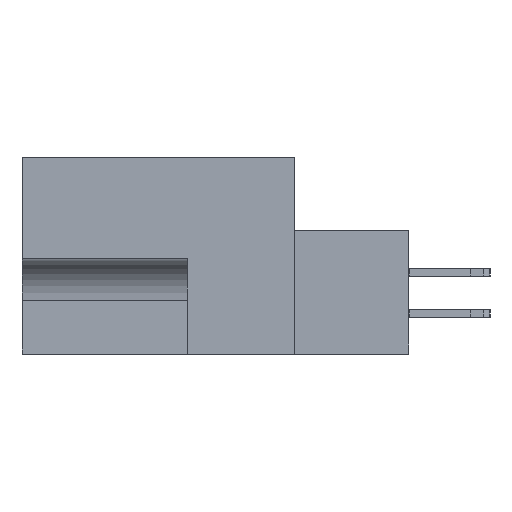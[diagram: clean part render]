
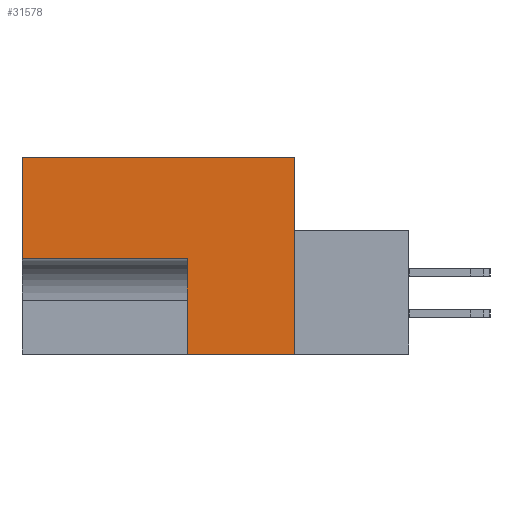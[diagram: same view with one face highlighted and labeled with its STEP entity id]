
A CAD part, left-side view. The second image highlights one B-rep face of the part: STEP entity #31578.
In plain terms, the highlighted planar face has unit normal (-1, 0, 0).
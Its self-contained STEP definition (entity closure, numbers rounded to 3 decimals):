
#2270 = FACE_OUTER_BOUND ( 'NONE', #22167, .T. ) ;
#3450 = ORIENTED_EDGE ( 'NONE', *, *, #34992, .F. ) ;
#3688 = DIRECTION ( 'NONE',  ( 0., 0., 1. ) ) ;
#6347 = DIRECTION ( 'NONE',  ( 1., 0., 0. ) ) ;
#6466 = EDGE_CURVE ( 'NONE', #24307, #24224, #41106, .T. ) ;
#7853 = ORIENTED_EDGE ( 'NONE', *, *, #50835, .F. ) ;
#8285 = CARTESIAN_POINT ( 'NONE',  ( 0., 0., -15.088 ) ) ;
#8500 = CARTESIAN_POINT ( 'NONE',  ( 0., 11.506, 0. ) ) ;
#8534 = LINE ( 'NONE', #10292, #43697 ) ;
#9744 = VERTEX_POINT ( 'NONE', #23225 ) ;
#9888 = VERTEX_POINT ( 'NONE', #8285 ) ;
#10292 = CARTESIAN_POINT ( 'NONE',  ( 0., 20.955, -15.088 ) ) ;
#10749 = DIRECTION ( 'NONE',  ( 0., 1., 0. ) ) ;
#11667 = VECTOR ( 'NONE', #10749, 1000. ) ;
#12361 = DIRECTION ( 'NONE',  ( 0., -1., 0. ) ) ;
#13448 = LINE ( 'NONE', #8500, #31034 ) ;
#13539 = VECTOR ( 'NONE', #51083, 1000. ) ;
#18238 = EDGE_CURVE ( 'NONE', #31724, #24307, #25372, .T. ) ;
#19044 = AXIS2_PLACEMENT_3D ( 'NONE', #30370, #6347, #50217 ) ;
#19798 = ORIENTED_EDGE ( 'NONE', *, *, #37607, .F. ) ;
#21826 = VECTOR ( 'NONE', #25233, 1000. ) ;
#22167 = EDGE_LOOP ( 'NONE', ( #51444, #3450, #19798, #7853, #46840, #31000 ) ) ;
#22314 = CARTESIAN_POINT ( 'NONE',  ( 0., 8.255, -7.772 ) ) ;
#22481 = EDGE_CURVE ( 'NONE', #9888, #31724, #31132, .T. ) ;
#23225 = CARTESIAN_POINT ( 'NONE',  ( 0., 20.955, 0. ) ) ;
#24224 = VERTEX_POINT ( 'NONE', #27553 ) ;
#24307 = VERTEX_POINT ( 'NONE', #36288 ) ;
#25233 = DIRECTION ( 'NONE',  ( 0., 0., -1. ) ) ;
#25372 = LINE ( 'NONE', #31723, #31031 ) ;
#26325 = PLANE ( 'NONE',  #19044 ) ;
#27216 = CARTESIAN_POINT ( 'NONE',  ( 0., 0., 0. ) ) ;
#27553 = CARTESIAN_POINT ( 'NONE',  ( 0., 20.955, -7.772 ) ) ;
#30370 = CARTESIAN_POINT ( 'NONE',  ( 0., 0., 0. ) ) ;
#30586 = CARTESIAN_POINT ( 'NONE',  ( 0., 8.255, -15.088 ) ) ;
#31000 = ORIENTED_EDGE ( 'NONE', *, *, #18238, .F. ) ;
#31031 = VECTOR ( 'NONE', #3688, 1000. ) ;
#31034 = VECTOR ( 'NONE', #12361, 1000. ) ;
#31132 = LINE ( 'NONE', #34360, #13539 ) ;
#31578 = ADVANCED_FACE ( 'NONE', ( #2270 ), #26325, .F. ) ;
#31723 = CARTESIAN_POINT ( 'NONE',  ( 0., 8.255, -15.088 ) ) ;
#31724 = VERTEX_POINT ( 'NONE', #30586 ) ;
#34096 = DIRECTION ( 'NONE',  ( 0., 0., 1. ) ) ;
#34360 = CARTESIAN_POINT ( 'NONE',  ( 0., -8.814, -15.088 ) ) ;
#34992 = EDGE_CURVE ( 'NONE', #51563, #9888, #51955, .T. ) ;
#36288 = CARTESIAN_POINT ( 'NONE',  ( 0., 8.255, -7.772 ) ) ;
#37607 = EDGE_CURVE ( 'NONE', #9744, #51563, #13448, .T. ) ;
#41106 = LINE ( 'NONE', #22314, #11667 ) ;
#43697 = VECTOR ( 'NONE', #34096, 1000. ) ;
#45082 = CARTESIAN_POINT ( 'NONE',  ( 0., 0., 0. ) ) ;
#46840 = ORIENTED_EDGE ( 'NONE', *, *, #6466, .F. ) ;
#50217 = DIRECTION ( 'NONE',  ( 0., 0., -1. ) ) ;
#50835 = EDGE_CURVE ( 'NONE', #24224, #9744, #8534, .T. ) ;
#51083 = DIRECTION ( 'NONE',  ( 0., 1., 0. ) ) ;
#51444 = ORIENTED_EDGE ( 'NONE', *, *, #22481, .F. ) ;
#51563 = VERTEX_POINT ( 'NONE', #27216 ) ;
#51955 = LINE ( 'NONE', #45082, #21826 ) ;
